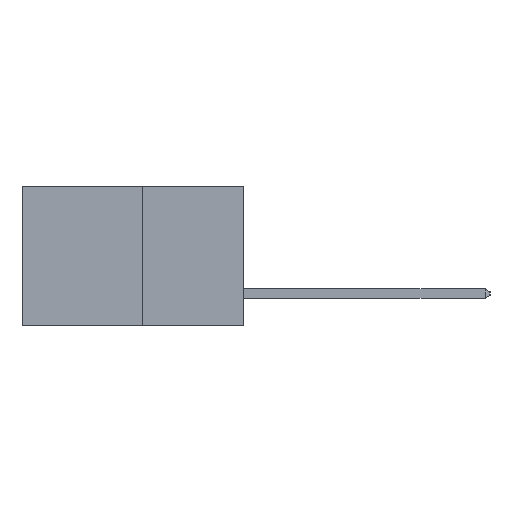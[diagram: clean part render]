
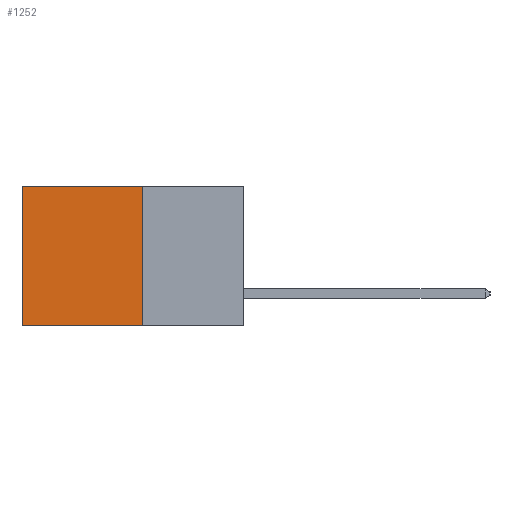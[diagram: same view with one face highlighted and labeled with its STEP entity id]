
A CAD part, left-side view. The second image highlights one B-rep face of the part: STEP entity #1252.
In plain terms, the highlighted planar face has unit normal (-1, 0, 0).
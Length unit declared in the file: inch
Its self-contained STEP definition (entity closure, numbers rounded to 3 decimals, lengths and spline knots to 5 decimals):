
#311 = VECTOR ( 'NONE', #16544, 39.37008 ) ;
#383 = EDGE_LOOP ( 'NONE', ( #5342, #7404, #9897, #15858 ) ) ;
#1252 = ADVANCED_FACE ( 'NONE', ( #8151 ), #8609, .F. ) ;
#1300 = AXIS2_PLACEMENT_3D ( 'NONE', #19533, #16061, #14972 ) ;
#3556 = EDGE_CURVE ( 'NONE', #5571, #9231, #8828, .T. ) ;
#4284 = LINE ( 'NONE', #14660, #13242 ) ;
#4443 = LINE ( 'NONE', #19364, #8430 ) ;
#5342 = ORIENTED_EDGE ( 'NONE', *, *, #3556, .T. ) ;
#5571 = VERTEX_POINT ( 'NONE', #17126 ) ;
#5894 = CARTESIAN_POINT ( 'NONE',  ( 0.277, 0.27, -0.37 ) ) ;
#6053 = LINE ( 'NONE', #20267, #18387 ) ;
#7342 = VERTEX_POINT ( 'NONE', #5894 ) ;
#7404 = ORIENTED_EDGE ( 'NONE', *, *, #7553, .F. ) ;
#7493 = EDGE_CURVE ( 'NONE', #17679, #5571, #6053, .T. ) ;
#7553 = EDGE_CURVE ( 'NONE', #7342, #9231, #4443, .T. ) ;
#8151 = FACE_OUTER_BOUND ( 'NONE', #383, .T. ) ;
#8430 = VECTOR ( 'NONE', #19278, 39.37008 ) ;
#8609 = PLANE ( 'NONE',  #1300 ) ;
#8828 = LINE ( 'NONE', #16905, #311 ) ;
#9231 = VERTEX_POINT ( 'NONE', #15805 ) ;
#9897 = ORIENTED_EDGE ( 'NONE', *, *, #10684, .F. ) ;
#10684 = EDGE_CURVE ( 'NONE', #17679, #7342, #4284, .T. ) ;
#13242 = VECTOR ( 'NONE', #21276, 39.37008 ) ;
#14660 = CARTESIAN_POINT ( 'NONE',  ( 0.277, 0.27, -0.37 ) ) ;
#14972 = DIRECTION ( 'NONE',  ( 0., 0., -1. ) ) ;
#15805 = CARTESIAN_POINT ( 'NONE',  ( 0.277, 0.59, -0.37 ) ) ;
#15858 = ORIENTED_EDGE ( 'NONE', *, *, #7493, .T. ) ;
#16061 = DIRECTION ( 'NONE',  ( 1., 0., 0. ) ) ;
#16466 = CARTESIAN_POINT ( 'NONE',  ( 0.277, 0.27, 0. ) ) ;
#16544 = DIRECTION ( 'NONE',  ( 0., 0., -1. ) ) ;
#16905 = CARTESIAN_POINT ( 'NONE',  ( 0.277, 0.59, -0.37 ) ) ;
#17126 = CARTESIAN_POINT ( 'NONE',  ( 0.277, 0.59, 0. ) ) ;
#17679 = VERTEX_POINT ( 'NONE', #16466 ) ;
#18387 = VECTOR ( 'NONE', #20156, 39.37008 ) ;
#19278 = DIRECTION ( 'NONE',  ( 0., 1., 0. ) ) ;
#19364 = CARTESIAN_POINT ( 'NONE',  ( 0.277, 0.27, -0.37 ) ) ;
#19533 = CARTESIAN_POINT ( 'NONE',  ( 0.277, 0.27, -0.37 ) ) ;
#20156 = DIRECTION ( 'NONE',  ( 0., 1., 0. ) ) ;
#20267 = CARTESIAN_POINT ( 'NONE',  ( 0.277, 0.27, 0. ) ) ;
#21276 = DIRECTION ( 'NONE',  ( 0., 0., -1. ) ) ;
